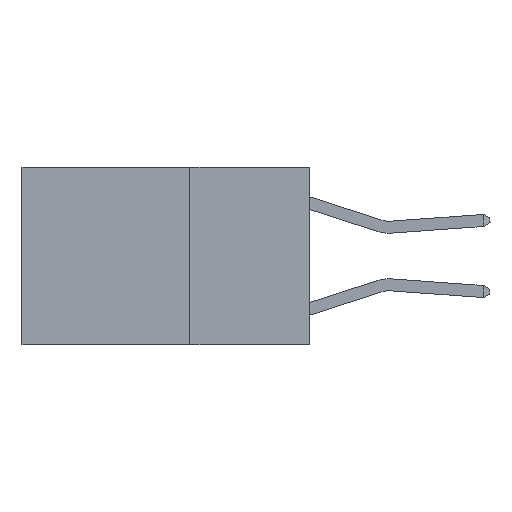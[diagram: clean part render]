
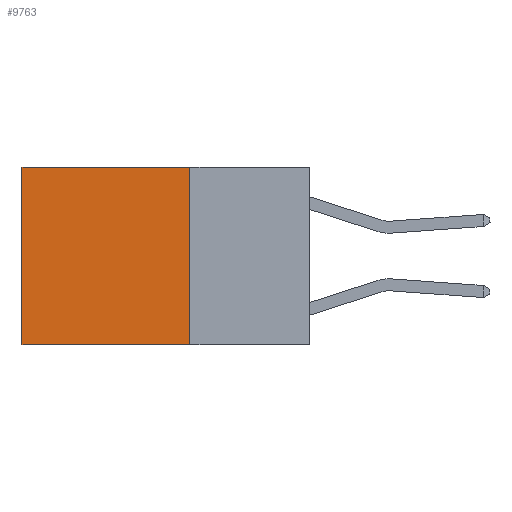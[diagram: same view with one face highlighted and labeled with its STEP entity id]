
A CAD part, left-side view. The second image highlights one B-rep face of the part: STEP entity #9763.
In plain terms, the highlighted planar face has unit normal (-1, 0, 0).
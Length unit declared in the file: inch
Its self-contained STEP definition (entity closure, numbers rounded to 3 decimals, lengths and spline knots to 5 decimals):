
#33 = VERTEX_POINT ( 'NONE', #6146 ) ;
#954 = DIRECTION ( 'NONE',  ( 0., 0., -1. ) ) ;
#1195 = DIRECTION ( 'NONE',  ( 0., 1., 0. ) ) ;
#1268 = EDGE_CURVE ( 'NONE', #33, #9821, #8099, .T. ) ;
#1325 = ORIENTED_EDGE ( 'NONE', *, *, #9567, .T. ) ;
#1632 = ORIENTED_EDGE ( 'NONE', *, *, #8365, .F. ) ;
#1644 = CARTESIAN_POINT ( 'NONE',  ( 0.2625, 0.6, -0.37 ) ) ;
#1854 = FACE_OUTER_BOUND ( 'NONE', #6970, .T. ) ;
#1950 = ORIENTED_EDGE ( 'NONE', *, *, #1268, .T. ) ;
#2730 = LINE ( 'NONE', #3897, #10234 ) ;
#2777 = CARTESIAN_POINT ( 'NONE',  ( 0.2625, 0.25, 0. ) ) ;
#3897 = CARTESIAN_POINT ( 'NONE',  ( 0.2625, 0.25, 0. ) ) ;
#3948 = ORIENTED_EDGE ( 'NONE', *, *, #7853, .F. ) ;
#4321 = VECTOR ( 'NONE', #9586, 39.37008 ) ;
#4885 = CARTESIAN_POINT ( 'NONE',  ( 0.2625, 0.25, -0.37 ) ) ;
#5192 = VECTOR ( 'NONE', #8291, 39.37008 ) ;
#5372 = LINE ( 'NONE', #8027, #10249 ) ;
#5746 = DIRECTION ( 'NONE',  ( 0., 0., -1. ) ) ;
#6146 = CARTESIAN_POINT ( 'NONE',  ( 0.2625, 0.25, 0. ) ) ;
#6970 = EDGE_LOOP ( 'NONE', ( #1325, #3948, #1632, #1950 ) ) ;
#7853 = EDGE_CURVE ( 'NONE', #8368, #12146, #5372, .T. ) ;
#8027 = CARTESIAN_POINT ( 'NONE',  ( 0.2625, 0.25, -0.37 ) ) ;
#8099 = LINE ( 'NONE', #10195, #5192 ) ;
#8291 = DIRECTION ( 'NONE',  ( 0., 1., 0. ) ) ;
#8327 = AXIS2_PLACEMENT_3D ( 'NONE', #2777, #11549, #5746 ) ;
#8365 = EDGE_CURVE ( 'NONE', #33, #8368, #2730, .T. ) ;
#8368 = VERTEX_POINT ( 'NONE', #4885 ) ;
#8608 = CARTESIAN_POINT ( 'NONE',  ( 0.2625, 0.6, 0. ) ) ;
#9567 = EDGE_CURVE ( 'NONE', #9821, #12146, #11761, .T. ) ;
#9586 = DIRECTION ( 'NONE',  ( 0., 0., -1. ) ) ;
#9691 = CARTESIAN_POINT ( 'NONE',  ( 0.2625, 0.6, 0. ) ) ;
#9763 = ADVANCED_FACE ( 'NONE', ( #1854 ), #12457, .F. ) ;
#9821 = VERTEX_POINT ( 'NONE', #9691 ) ;
#10195 = CARTESIAN_POINT ( 'NONE',  ( 0.2625, 0.25, 0. ) ) ;
#10234 = VECTOR ( 'NONE', #954, 39.37008 ) ;
#10249 = VECTOR ( 'NONE', #1195, 39.37008 ) ;
#11549 = DIRECTION ( 'NONE',  ( 1., 0., 0. ) ) ;
#11761 = LINE ( 'NONE', #8608, #4321 ) ;
#12146 = VERTEX_POINT ( 'NONE', #1644 ) ;
#12457 = PLANE ( 'NONE',  #8327 ) ;
